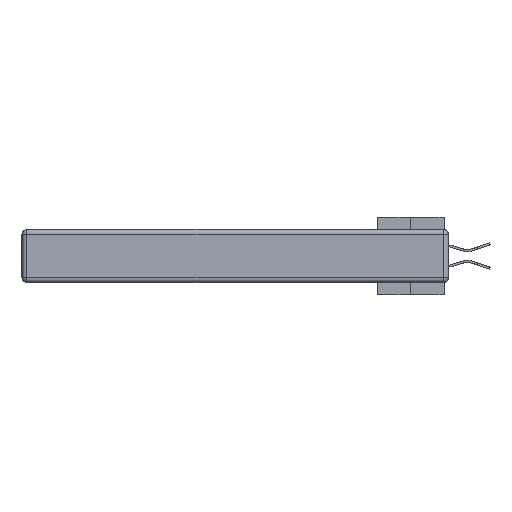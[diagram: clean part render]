
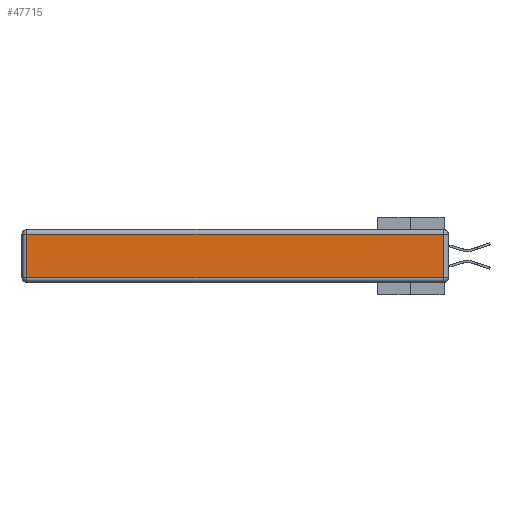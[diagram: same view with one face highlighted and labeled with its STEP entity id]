
A CAD part, left-side view. The second image highlights one B-rep face of the part: STEP entity #47715.
In plain terms, the highlighted planar face has unit normal (-1, 0, 0).
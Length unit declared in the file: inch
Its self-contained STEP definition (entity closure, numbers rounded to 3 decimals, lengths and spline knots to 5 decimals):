
#606 = EDGE_CURVE ( 'NONE', #37660, #18039, #45086, .T. ) ;
#620 = DIRECTION ( 'NONE',  ( 0., 0., 1. ) ) ;
#1983 = EDGE_CURVE ( 'NONE', #4910, #37660, #5269, .T. ) ;
#2813 = LINE ( 'NONE', #14775, #24400 ) ;
#3676 = DIRECTION ( 'NONE',  ( -1., 0., 0. ) ) ;
#4316 = CARTESIAN_POINT ( 'NONE',  ( 0., 2.72, -0.03 ) ) ;
#4910 = VERTEX_POINT ( 'NONE', #8291 ) ;
#5269 = LINE ( 'NONE', #7546, #10669 ) ;
#5559 = ORIENTED_EDGE ( 'NONE', *, *, #49506, .T. ) ;
#6583 = CARTESIAN_POINT ( 'NONE',  ( 0., 0.03, -0.343 ) ) ;
#7546 = CARTESIAN_POINT ( 'NONE',  ( 0., 2.75, -0.03 ) ) ;
#8188 = CARTESIAN_POINT ( 'NONE',  ( 0., 0., -0.343 ) ) ;
#8291 = CARTESIAN_POINT ( 'NONE',  ( 0., 0.03, -0.03 ) ) ;
#9560 = LINE ( 'NONE', #6583, #30590 ) ;
#10368 = AXIS2_PLACEMENT_3D ( 'NONE', #8188, #3676, #620 ) ;
#10669 = VECTOR ( 'NONE', #14971, 39.37008 ) ;
#12492 = EDGE_CURVE ( 'NONE', #21050, #4910, #9560, .T. ) ;
#13745 = FACE_OUTER_BOUND ( 'NONE', #32523, .T. ) ;
#14775 = CARTESIAN_POINT ( 'NONE',  ( 0., 0., -0.313 ) ) ;
#14971 = DIRECTION ( 'NONE',  ( 0., 1., 0. ) ) ;
#16919 = ORIENTED_EDGE ( 'NONE', *, *, #606, .T. ) ;
#18039 = VERTEX_POINT ( 'NONE', #24254 ) ;
#18894 = DIRECTION ( 'NONE',  ( 0., 0., -1. ) ) ;
#21050 = VERTEX_POINT ( 'NONE', #42876 ) ;
#23612 = PLANE ( 'NONE',  #10368 ) ;
#24254 = CARTESIAN_POINT ( 'NONE',  ( 0., 2.72, -0.313 ) ) ;
#24400 = VECTOR ( 'NONE', #26334, 39.37008 ) ;
#26334 = DIRECTION ( 'NONE',  ( 0., -1., 0. ) ) ;
#29743 = DIRECTION ( 'NONE',  ( 0., 0., 1. ) ) ;
#30590 = VECTOR ( 'NONE', #29743, 39.37008 ) ;
#32523 = EDGE_LOOP ( 'NONE', ( #5559, #35321, #39127, #16919 ) ) ;
#34915 = VECTOR ( 'NONE', #18894, 39.37008 ) ;
#35321 = ORIENTED_EDGE ( 'NONE', *, *, #12492, .T. ) ;
#37660 = VERTEX_POINT ( 'NONE', #4316 ) ;
#38394 = CARTESIAN_POINT ( 'NONE',  ( 0., 2.72, -0.343 ) ) ;
#39127 = ORIENTED_EDGE ( 'NONE', *, *, #1983, .T. ) ;
#42876 = CARTESIAN_POINT ( 'NONE',  ( 0., 0.03, -0.313 ) ) ;
#45086 = LINE ( 'NONE', #38394, #34915 ) ;
#47715 = ADVANCED_FACE ( 'NONE', ( #13745 ), #23612, .T. ) ;
#49506 = EDGE_CURVE ( 'NONE', #18039, #21050, #2813, .T. ) ;
